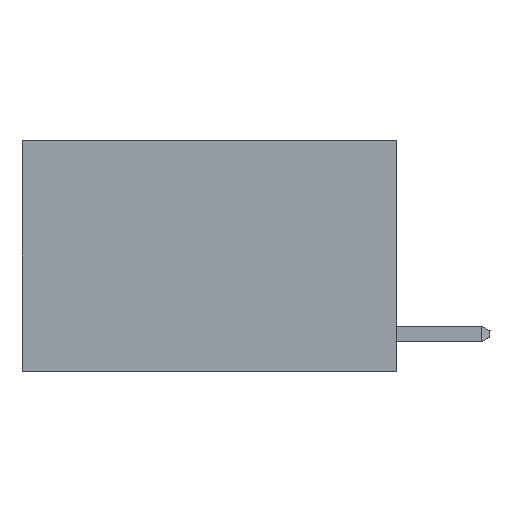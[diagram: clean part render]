
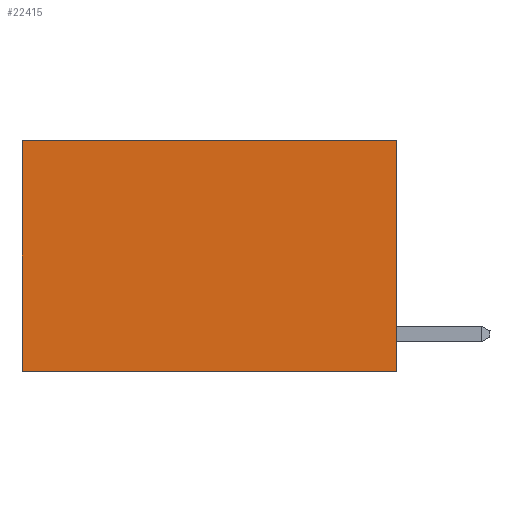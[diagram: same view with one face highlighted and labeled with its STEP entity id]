
A CAD part, left-side view. The second image highlights one B-rep face of the part: STEP entity #22415.
In plain terms, the highlighted planar face has unit normal (-1, 0, 0).
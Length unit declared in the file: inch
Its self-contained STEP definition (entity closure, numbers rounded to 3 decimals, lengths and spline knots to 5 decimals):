
#1892 = CARTESIAN_POINT ( 'NONE',  ( 0.2625, 0., 0. ) ) ;
#1899 = VERTEX_POINT ( 'NONE', #23281 ) ;
#2051 = CARTESIAN_POINT ( 'NONE',  ( 0.2625, 0.6, 0. ) ) ;
#3592 = DIRECTION ( 'NONE',  ( 1., 0., 0. ) ) ;
#3864 = PLANE ( 'NONE',  #23600 ) ;
#3932 = VECTOR ( 'NONE', #24480, 39.37008 ) ;
#3945 = CARTESIAN_POINT ( 'NONE',  ( 0.2625, 0., 0. ) ) ;
#4229 = CARTESIAN_POINT ( 'NONE',  ( 0.2625, 0.6, 0. ) ) ;
#5007 = FACE_OUTER_BOUND ( 'NONE', #19377, .T. ) ;
#5781 = DIRECTION ( 'NONE',  ( 0., 0., -1. ) ) ;
#6259 = ORIENTED_EDGE ( 'NONE', *, *, #8480, .T. ) ;
#8480 = EDGE_CURVE ( 'NONE', #13517, #1899, #23360, .T. ) ;
#9063 = VECTOR ( 'NONE', #12286, 39.37008 ) ;
#9196 = ORIENTED_EDGE ( 'NONE', *, *, #16481, .F. ) ;
#9451 = EDGE_CURVE ( 'NONE', #23289, #1899, #18932, .T. ) ;
#10879 = ORIENTED_EDGE ( 'NONE', *, *, #9451, .F. ) ;
#12286 = DIRECTION ( 'NONE',  ( 0., 1., 0. ) ) ;
#12883 = CARTESIAN_POINT ( 'NONE',  ( 0.2625, 0., -0.37 ) ) ;
#12950 = EDGE_CURVE ( 'NONE', #22501, #13517, #24273, .T. ) ;
#13351 = ORIENTED_EDGE ( 'NONE', *, *, #12950, .T. ) ;
#13517 = VERTEX_POINT ( 'NONE', #2051 ) ;
#14081 = VECTOR ( 'NONE', #24778, 39.37008 ) ;
#15646 = VECTOR ( 'NONE', #5781, 39.37008 ) ;
#16421 = CARTESIAN_POINT ( 'NONE',  ( 0.2625, 0., 0. ) ) ;
#16481 = EDGE_CURVE ( 'NONE', #22501, #23289, #26044, .T. ) ;
#18115 = DIRECTION ( 'NONE',  ( 0., 0., -1. ) ) ;
#18521 = CARTESIAN_POINT ( 'NONE',  ( 0.2625, 0., 0. ) ) ;
#18932 = LINE ( 'NONE', #26244, #14081 ) ;
#19377 = EDGE_LOOP ( 'NONE', ( #6259, #10879, #9196, #13351 ) ) ;
#22415 = ADVANCED_FACE ( 'NONE', ( #5007 ), #3864, .F. ) ;
#22501 = VERTEX_POINT ( 'NONE', #1892 ) ;
#23281 = CARTESIAN_POINT ( 'NONE',  ( 0.2625, 0.6, -0.37 ) ) ;
#23289 = VERTEX_POINT ( 'NONE', #12883 ) ;
#23360 = LINE ( 'NONE', #4229, #3932 ) ;
#23600 = AXIS2_PLACEMENT_3D ( 'NONE', #3945, #3592, #18115 ) ;
#24273 = LINE ( 'NONE', #18521, #9063 ) ;
#24480 = DIRECTION ( 'NONE',  ( 0., 0., -1. ) ) ;
#24778 = DIRECTION ( 'NONE',  ( 0., 1., 0. ) ) ;
#26044 = LINE ( 'NONE', #16421, #15646 ) ;
#26244 = CARTESIAN_POINT ( 'NONE',  ( 0.2625, 0., -0.37 ) ) ;
